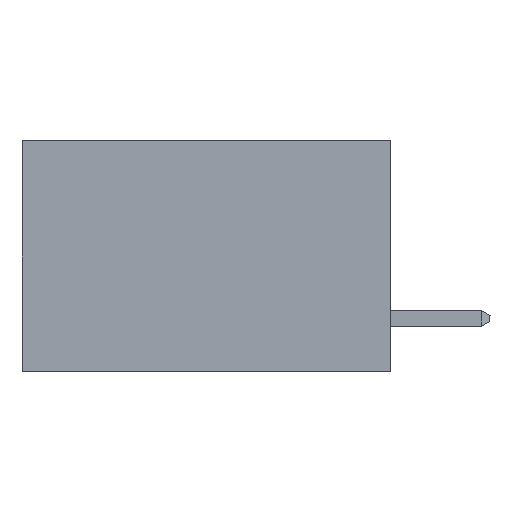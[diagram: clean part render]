
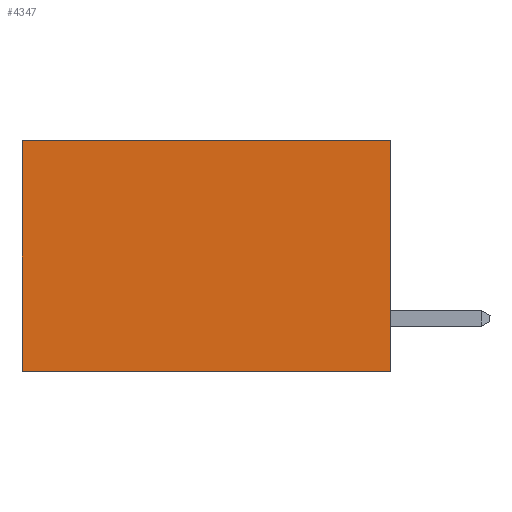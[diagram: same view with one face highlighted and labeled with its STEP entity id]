
A CAD part, left-side view. The second image highlights one B-rep face of the part: STEP entity #4347.
In plain terms, the highlighted planar face has unit normal (-1, 0, 0).
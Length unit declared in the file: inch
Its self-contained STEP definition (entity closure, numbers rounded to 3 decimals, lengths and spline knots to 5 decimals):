
#648 = CARTESIAN_POINT ( 'NONE',  ( 0.277, 0., -0.37 ) ) ;
#679 = CARTESIAN_POINT ( 'NONE',  ( 0.277, 0., -0.37 ) ) ;
#765 = ORIENTED_EDGE ( 'NONE', *, *, #9879, .T. ) ;
#849 = EDGE_CURVE ( 'NONE', #2078, #6580, #5026, .T. ) ;
#889 = DIRECTION ( 'NONE',  ( 0., 0., -1. ) ) ;
#1678 = LINE ( 'NONE', #6914, #10434 ) ;
#2078 = VERTEX_POINT ( 'NONE', #5194 ) ;
#2930 = ORIENTED_EDGE ( 'NONE', *, *, #9737, .T. ) ;
#3099 = DIRECTION ( 'NONE',  ( 0., 0., -1. ) ) ;
#3101 = DIRECTION ( 'NONE',  ( 1., 0., 0. ) ) ;
#3185 = PLANE ( 'NONE',  #4187 ) ;
#3298 = CARTESIAN_POINT ( 'NONE',  ( 0.277, 0., -0.37 ) ) ;
#3814 = CARTESIAN_POINT ( 'NONE',  ( 0.277, 0., 0. ) ) ;
#4187 = AXIS2_PLACEMENT_3D ( 'NONE', #3298, #3101, #3099 ) ;
#4347 = ADVANCED_FACE ( 'NONE', ( #10724 ), #3185, .F. ) ;
#4730 = LINE ( 'NONE', #3814, #6612 ) ;
#5026 = LINE ( 'NONE', #679, #6677 ) ;
#5181 = ORIENTED_EDGE ( 'NONE', *, *, #5679, .F. ) ;
#5194 = CARTESIAN_POINT ( 'NONE',  ( 0.277, 0., 0. ) ) ;
#5550 = DIRECTION ( 'NONE',  ( 0., 1., 0. ) ) ;
#5679 = EDGE_CURVE ( 'NONE', #6580, #5795, #10032, .T. ) ;
#5754 = CARTESIAN_POINT ( 'NONE',  ( 0.277, 0., -0.37 ) ) ;
#5795 = VERTEX_POINT ( 'NONE', #10955 ) ;
#6580 = VERTEX_POINT ( 'NONE', #648 ) ;
#6612 = VECTOR ( 'NONE', #7095, 39.37008 ) ;
#6677 = VECTOR ( 'NONE', #889, 39.37008 ) ;
#6914 = CARTESIAN_POINT ( 'NONE',  ( 0.277, 0.59, -0.37 ) ) ;
#7095 = DIRECTION ( 'NONE',  ( 0., 1., 0. ) ) ;
#7138 = EDGE_LOOP ( 'NONE', ( #2930, #5181, #7357, #765 ) ) ;
#7231 = CARTESIAN_POINT ( 'NONE',  ( 0.277, 0.59, 0. ) ) ;
#7357 = ORIENTED_EDGE ( 'NONE', *, *, #849, .F. ) ;
#7784 = VECTOR ( 'NONE', #5550, 39.37008 ) ;
#8510 = VERTEX_POINT ( 'NONE', #7231 ) ;
#9482 = DIRECTION ( 'NONE',  ( 0., 0., -1. ) ) ;
#9737 = EDGE_CURVE ( 'NONE', #8510, #5795, #1678, .T. ) ;
#9879 = EDGE_CURVE ( 'NONE', #2078, #8510, #4730, .T. ) ;
#10032 = LINE ( 'NONE', #5754, #7784 ) ;
#10434 = VECTOR ( 'NONE', #9482, 39.37008 ) ;
#10724 = FACE_OUTER_BOUND ( 'NONE', #7138, .T. ) ;
#10955 = CARTESIAN_POINT ( 'NONE',  ( 0.277, 0.59, -0.37 ) ) ;
